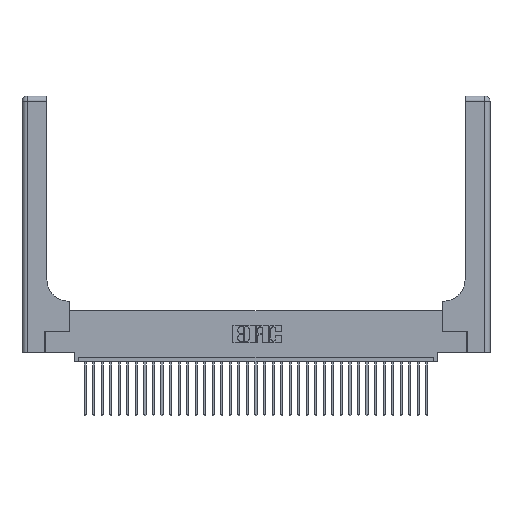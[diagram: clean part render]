
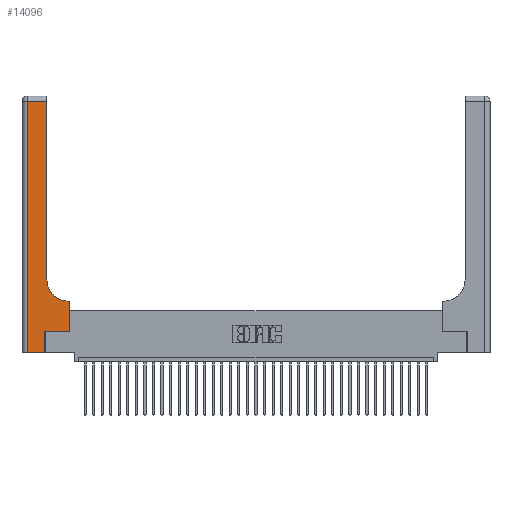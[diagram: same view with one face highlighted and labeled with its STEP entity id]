
A CAD part, top view. The second image highlights one B-rep face of the part: STEP entity #14096.
In plain terms, the highlighted planar face has unit normal (0, 0, 1).
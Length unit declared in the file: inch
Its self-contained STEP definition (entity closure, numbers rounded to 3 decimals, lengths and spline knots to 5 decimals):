
#45 = VECTOR ( 'NONE', #31809, 39.37008 ) ;
#235 = DIRECTION ( 'NONE',  ( 1., 0., 0. ) ) ;
#577 = EDGE_CURVE ( 'NONE', #16179, #23042, #11615, .T. ) ;
#618 = CARTESIAN_POINT ( 'NONE',  ( 0., 3., 0.37 ) ) ;
#987 = CARTESIAN_POINT ( 'NONE',  ( 0., 0., 0.37 ) ) ;
#1120 = EDGE_LOOP ( 'NONE', ( #33917, #24733, #35496, #10901, #17422, #1968, #31192, #35297, #7566 ) ) ;
#1122 = CARTESIAN_POINT ( 'NONE',  ( 0.5585, 0.25, 0.37 ) ) ;
#1787 = CARTESIAN_POINT ( 'NONE',  ( 0.5415, 0.85, 0.37 ) ) ;
#1894 = CARTESIAN_POINT ( 'NONE',  ( 0.06, 2.94, 0.37 ) ) ;
#1968 = ORIENTED_EDGE ( 'NONE', *, *, #3591, .T. ) ;
#2026 = DIRECTION ( 'NONE',  ( 0., 0., -1. ) ) ;
#2253 = CARTESIAN_POINT ( 'NONE',  ( 0.06, 0., 0.37 ) ) ;
#2619 = DIRECTION ( 'NONE',  ( -1., 0., 0. ) ) ;
#2689 = DIRECTION ( 'NONE',  ( -1., 0., 0. ) ) ;
#2957 = VERTEX_POINT ( 'NONE', #1894 ) ;
#3591 = EDGE_CURVE ( 'NONE', #16294, #33098, #14535, .T. ) ;
#4309 = CARTESIAN_POINT ( 'NONE',  ( 0.269, 0.25, 0.37 ) ) ;
#4362 = DIRECTION ( 'NONE',  ( -1., 0., 0. ) ) ;
#5382 = EDGE_CURVE ( 'NONE', #2957, #23403, #22709, .T. ) ;
#6567 = DIRECTION ( 'NONE',  ( 0., 1., 0. ) ) ;
#6604 = EDGE_CURVE ( 'NONE', #25244, #2957, #25460, .T. ) ;
#7566 = ORIENTED_EDGE ( 'NONE', *, *, #29301, .T. ) ;
#9046 = EDGE_CURVE ( 'NONE', #15291, #16294, #12597, .T. ) ;
#10343 = CIRCLE ( 'NONE', #28989, 0.25 ) ;
#10901 = ORIENTED_EDGE ( 'NONE', *, *, #27219, .T. ) ;
#11615 = LINE ( 'NONE', #13762, #26467 ) ;
#12156 = LINE ( 'NONE', #29807, #22234 ) ;
#12177 = CARTESIAN_POINT ( 'NONE',  ( 0.5585, 0.6, 0.37 ) ) ;
#12552 = PLANE ( 'NONE',  #15591 ) ;
#12597 = LINE ( 'NONE', #25344, #22676 ) ;
#12629 = VECTOR ( 'NONE', #26916, 39.37008 ) ;
#12773 = VECTOR ( 'NONE', #4362, 39.37008 ) ;
#13762 = CARTESIAN_POINT ( 'NONE',  ( 0.2915, 0.6, 0.37 ) ) ;
#14096 = ADVANCED_FACE ( 'NONE', ( #19587 ), #12552, .F. ) ;
#14535 = LINE ( 'NONE', #4309, #45 ) ;
#14627 = VECTOR ( 'NONE', #6567, 39.37008 ) ;
#15254 = VECTOR ( 'NONE', #235, 39.37008 ) ;
#15291 = VERTEX_POINT ( 'NONE', #25005 ) ;
#15591 = AXIS2_PLACEMENT_3D ( 'NONE', #618, #20715, #2619 ) ;
#15886 = CARTESIAN_POINT ( 'NONE',  ( 0.2915, 2.94, 0.37 ) ) ;
#16179 = VERTEX_POINT ( 'NONE', #12177 ) ;
#16294 = VERTEX_POINT ( 'NONE', #24140 ) ;
#16930 = VERTEX_POINT ( 'NONE', #17644 ) ;
#17422 = ORIENTED_EDGE ( 'NONE', *, *, #9046, .T. ) ;
#17581 = CARTESIAN_POINT ( 'NONE',  ( 0.2915, 3., 0.37 ) ) ;
#17644 = CARTESIAN_POINT ( 'NONE',  ( 0.2915, 0.85, 0.37 ) ) ;
#17876 = CARTESIAN_POINT ( 'NONE',  ( 0.5415, 0.6, 0.37 ) ) ;
#18183 = DIRECTION ( 'NONE',  ( 0., 1., 0. ) ) ;
#18948 = LINE ( 'NONE', #17581, #14627 ) ;
#19587 = FACE_OUTER_BOUND ( 'NONE', #1120, .T. ) ;
#19606 = LINE ( 'NONE', #987, #15254 ) ;
#19969 = DIRECTION ( 'NONE',  ( 0., 1., 0. ) ) ;
#20715 = DIRECTION ( 'NONE',  ( 0., 0., -1. ) ) ;
#21632 = DIRECTION ( 'NONE',  ( 1., 0., 0. ) ) ;
#22234 = VECTOR ( 'NONE', #18183, 39.37008 ) ;
#22676 = VECTOR ( 'NONE', #19969, 39.37008 ) ;
#22709 = LINE ( 'NONE', #29863, #12629 ) ;
#23042 = VERTEX_POINT ( 'NONE', #17876 ) ;
#23403 = VERTEX_POINT ( 'NONE', #2253 ) ;
#24140 = CARTESIAN_POINT ( 'NONE',  ( 0.269, 0.25, 0.37 ) ) ;
#24733 = ORIENTED_EDGE ( 'NONE', *, *, #6604, .T. ) ;
#25005 = CARTESIAN_POINT ( 'NONE',  ( 0.269, 0., 0.37 ) ) ;
#25244 = VERTEX_POINT ( 'NONE', #15886 ) ;
#25344 = CARTESIAN_POINT ( 'NONE',  ( 0.269, 0., 0.37 ) ) ;
#25460 = LINE ( 'NONE', #29933, #12773 ) ;
#26467 = VECTOR ( 'NONE', #2689, 39.37008 ) ;
#26916 = DIRECTION ( 'NONE',  ( 0., -1., 0. ) ) ;
#27219 = EDGE_CURVE ( 'NONE', #23403, #15291, #19606, .T. ) ;
#28451 = EDGE_CURVE ( 'NONE', #33098, #16179, #12156, .T. ) ;
#28989 = AXIS2_PLACEMENT_3D ( 'NONE', #1787, #2026, #21632 ) ;
#29301 = EDGE_CURVE ( 'NONE', #23042, #16930, #10343, .T. ) ;
#29807 = CARTESIAN_POINT ( 'NONE',  ( 0.5585, 0.25, 0.37 ) ) ;
#29863 = CARTESIAN_POINT ( 'NONE',  ( 0.06, 3., 0.37 ) ) ;
#29933 = CARTESIAN_POINT ( 'NONE',  ( 0., 2.94, 0.37 ) ) ;
#31192 = ORIENTED_EDGE ( 'NONE', *, *, #28451, .T. ) ;
#31809 = DIRECTION ( 'NONE',  ( 1., 0., 0. ) ) ;
#33098 = VERTEX_POINT ( 'NONE', #1122 ) ;
#33917 = ORIENTED_EDGE ( 'NONE', *, *, #35126, .T. ) ;
#35126 = EDGE_CURVE ( 'NONE', #16930, #25244, #18948, .T. ) ;
#35297 = ORIENTED_EDGE ( 'NONE', *, *, #577, .T. ) ;
#35496 = ORIENTED_EDGE ( 'NONE', *, *, #5382, .T. ) ;
